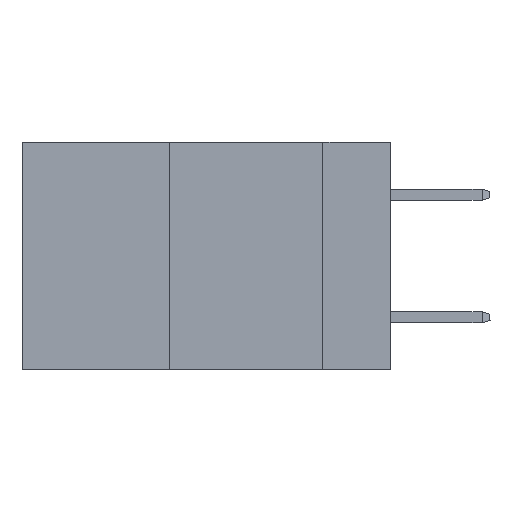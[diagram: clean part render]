
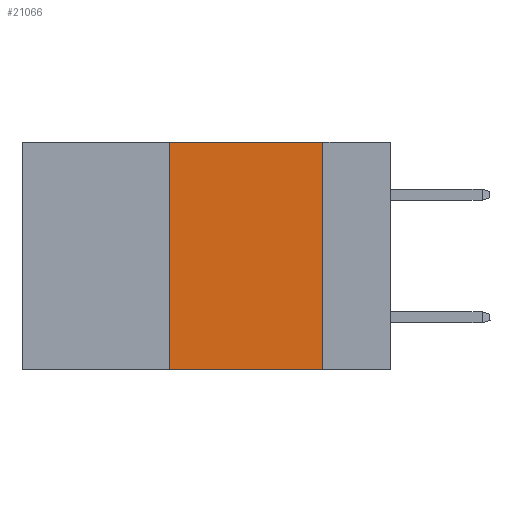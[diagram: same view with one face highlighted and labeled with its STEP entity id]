
A CAD part, left-side view. The second image highlights one B-rep face of the part: STEP entity #21066.
In plain terms, the highlighted planar face has unit normal (-1, 0, 0).
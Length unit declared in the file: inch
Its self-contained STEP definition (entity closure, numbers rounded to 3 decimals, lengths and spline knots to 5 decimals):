
#215 = EDGE_CURVE ( 'NONE', #21780, #3121, #15835, .T. ) ;
#1004 = CARTESIAN_POINT ( 'NONE',  ( 0., 0.6, -0.37 ) ) ;
#1461 = CARTESIAN_POINT ( 'NONE',  ( 0., 0.36, 0. ) ) ;
#1914 = LINE ( 'NONE', #1004, #12248 ) ;
#1922 = EDGE_CURVE ( 'NONE', #16562, #3121, #1914, .T. ) ;
#2609 = DIRECTION ( 'NONE',  ( 0., -1., 0. ) ) ;
#2863 = CARTESIAN_POINT ( 'NONE',  ( 0., 0.6, 0. ) ) ;
#3121 = VERTEX_POINT ( 'NONE', #12658 ) ;
#3753 = ORIENTED_EDGE ( 'NONE', *, *, #215, .F. ) ;
#4012 = VERTEX_POINT ( 'NONE', #5394 ) ;
#5394 = CARTESIAN_POINT ( 'NONE',  ( 0., 0.36, 0. ) ) ;
#9420 = DIRECTION ( 'NONE',  ( 0., 0., 1. ) ) ;
#9926 = EDGE_LOOP ( 'NONE', ( #3753, #15077, #13731, #23358 ) ) ;
#12248 = VECTOR ( 'NONE', #2609, 39.37008 ) ;
#12658 = CARTESIAN_POINT ( 'NONE',  ( 0., 0.11, -0.37 ) ) ;
#12821 = CARTESIAN_POINT ( 'NONE',  ( 0., 0.11, 0. ) ) ;
#13025 = LINE ( 'NONE', #17052, #23092 ) ;
#13731 = ORIENTED_EDGE ( 'NONE', *, *, #19357, .F. ) ;
#15077 = ORIENTED_EDGE ( 'NONE', *, *, #16369, .F. ) ;
#15122 = AXIS2_PLACEMENT_3D ( 'NONE', #2863, #17083, #23144 ) ;
#15136 = PLANE ( 'NONE',  #15122 ) ;
#15835 = LINE ( 'NONE', #12821, #21795 ) ;
#16369 = EDGE_CURVE ( 'NONE', #4012, #21780, #13025, .T. ) ;
#16562 = VERTEX_POINT ( 'NONE', #25646 ) ;
#17052 = CARTESIAN_POINT ( 'NONE',  ( 0., 0.6, 0. ) ) ;
#17083 = DIRECTION ( 'NONE',  ( 1., 0., 0. ) ) ;
#19244 = DIRECTION ( 'NONE',  ( 0., -1., 0. ) ) ;
#19357 = EDGE_CURVE ( 'NONE', #16562, #4012, #21619, .T. ) ;
#20658 = VECTOR ( 'NONE', #9420, 39.37008 ) ;
#21066 = ADVANCED_FACE ( 'NONE', ( #22784 ), #15136, .F. ) ;
#21619 = LINE ( 'NONE', #1461, #20658 ) ;
#21780 = VERTEX_POINT ( 'NONE', #25675 ) ;
#21795 = VECTOR ( 'NONE', #24936, 39.37008 ) ;
#22784 = FACE_OUTER_BOUND ( 'NONE', #9926, .T. ) ;
#23092 = VECTOR ( 'NONE', #19244, 39.37008 ) ;
#23144 = DIRECTION ( 'NONE',  ( 0., 0., -1. ) ) ;
#23358 = ORIENTED_EDGE ( 'NONE', *, *, #1922, .T. ) ;
#24936 = DIRECTION ( 'NONE',  ( 0., 0., -1. ) ) ;
#25646 = CARTESIAN_POINT ( 'NONE',  ( 0., 0.36, -0.37 ) ) ;
#25675 = CARTESIAN_POINT ( 'NONE',  ( 0., 0.11, 0. ) ) ;
